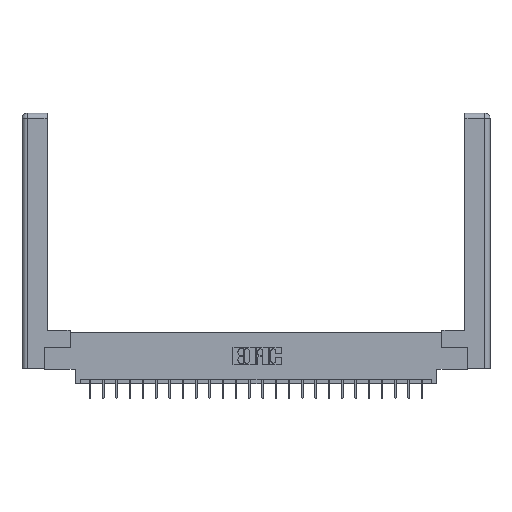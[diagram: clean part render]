
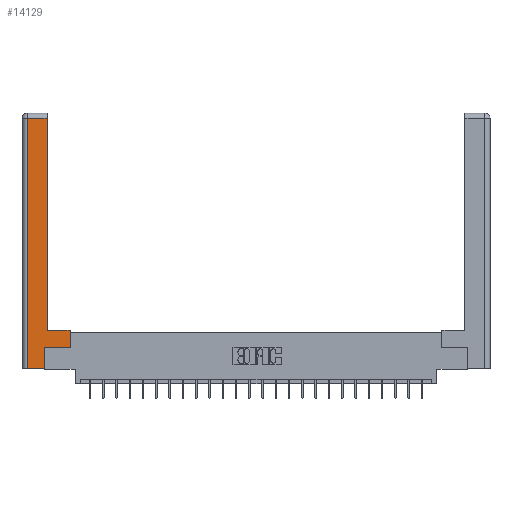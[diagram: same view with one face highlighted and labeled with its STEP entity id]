
A CAD part, top view. The second image highlights one B-rep face of the part: STEP entity #14129.
In plain terms, the highlighted planar face has unit normal (0, 0, 1).
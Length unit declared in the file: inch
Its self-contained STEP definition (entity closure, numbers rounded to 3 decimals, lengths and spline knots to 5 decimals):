
#980 = VERTEX_POINT ( 'NONE', #5465 ) ;
#1753 = CARTESIAN_POINT ( 'NONE',  ( 0.265, 0.245, 0. ) ) ;
#2010 = DIRECTION ( 'NONE',  ( 0., 1., 0. ) ) ;
#2089 = CARTESIAN_POINT ( 'NONE',  ( 0.265, 0.245, 0. ) ) ;
#2194 = LINE ( 'NONE', #23562, #3398 ) ;
#2288 = VERTEX_POINT ( 'NONE', #1753 ) ;
#2448 = DIRECTION ( 'NONE',  ( 1., 0., 0. ) ) ;
#2698 = LINE ( 'NONE', #21535, #18513 ) ;
#2741 = DIRECTION ( 'NONE',  ( 0., 0., -1. ) ) ;
#2962 = LINE ( 'NONE', #2089, #20273 ) ;
#3398 = VECTOR ( 'NONE', #2448, 39.37008 ) ;
#3611 = EDGE_CURVE ( 'NONE', #980, #16728, #10572, .T. ) ;
#3645 = ORIENTED_EDGE ( 'NONE', *, *, #22817, .T. ) ;
#3765 = ORIENTED_EDGE ( 'NONE', *, *, #8589, .T. ) ;
#4006 = LINE ( 'NONE', #23891, #23438 ) ;
#4472 = VECTOR ( 'NONE', #15790, 39.37008 ) ;
#5104 = ORIENTED_EDGE ( 'NONE', *, *, #24784, .T. ) ;
#5377 = EDGE_CURVE ( 'NONE', #16149, #980, #4006, .T. ) ;
#5465 = CARTESIAN_POINT ( 'NONE',  ( 0.295, 2.94, 0. ) ) ;
#5997 = CARTESIAN_POINT ( 'NONE',  ( 0.0615, 2.94, 0. ) ) ;
#6437 = CARTESIAN_POINT ( 'NONE',  ( 0., 0., 0. ) ) ;
#8413 = ORIENTED_EDGE ( 'NONE', *, *, #18346, .T. ) ;
#8589 = EDGE_CURVE ( 'NONE', #23346, #13900, #23147, .T. ) ;
#8873 = VECTOR ( 'NONE', #22036, 39.37008 ) ;
#10470 = DIRECTION ( 'NONE',  ( -1., 0., 0. ) ) ;
#10572 = LINE ( 'NONE', #5997, #4472 ) ;
#10596 = ORIENTED_EDGE ( 'NONE', *, *, #5377, .T. ) ;
#10843 = CARTESIAN_POINT ( 'NONE',  ( 0.295, 0.45, 0. ) ) ;
#11205 = EDGE_CURVE ( 'NONE', #2288, #22626, #2194, .T. ) ;
#11314 = DIRECTION ( 'NONE',  ( 0., -1., 0. ) ) ;
#11796 = VECTOR ( 'NONE', #11314, 39.37008 ) ;
#11833 = DIRECTION ( 'NONE',  ( 0., 1., 0. ) ) ;
#12417 = CARTESIAN_POINT ( 'NONE',  ( 0.265, 0., 0. ) ) ;
#12524 = ORIENTED_EDGE ( 'NONE', *, *, #14390, .T. ) ;
#13453 = CARTESIAN_POINT ( 'NONE',  ( 0.0615, 2.94, 0. ) ) ;
#13900 = VERTEX_POINT ( 'NONE', #23189 ) ;
#14129 = ADVANCED_FACE ( 'NONE', ( #18142 ), #16168, .F. ) ;
#14267 = DIRECTION ( 'NONE',  ( 0., 1., 0. ) ) ;
#14390 = EDGE_CURVE ( 'NONE', #13900, #2288, #2962, .T. ) ;
#14585 = AXIS2_PLACEMENT_3D ( 'NONE', #6437, #2741, #10470 ) ;
#14938 = EDGE_LOOP ( 'NONE', ( #10596, #19105, #5104, #3765, #12524, #23354, #8413, #3645 ) ) ;
#15790 = DIRECTION ( 'NONE',  ( -1., 0., 0. ) ) ;
#15851 = LINE ( 'NONE', #10843, #20388 ) ;
#16149 = VERTEX_POINT ( 'NONE', #21591 ) ;
#16168 = PLANE ( 'NONE',  #14585 ) ;
#16504 = VERTEX_POINT ( 'NONE', #24861 ) ;
#16609 = CARTESIAN_POINT ( 'NONE',  ( 0.565, 0.245, 0. ) ) ;
#16728 = VERTEX_POINT ( 'NONE', #13453 ) ;
#17296 = LINE ( 'NONE', #20960, #11796 ) ;
#18142 = FACE_OUTER_BOUND ( 'NONE', #14938, .T. ) ;
#18346 = EDGE_CURVE ( 'NONE', #22626, #16504, #2698, .T. ) ;
#18513 = VECTOR ( 'NONE', #11833, 39.37008 ) ;
#19105 = ORIENTED_EDGE ( 'NONE', *, *, #3611, .T. ) ;
#20273 = VECTOR ( 'NONE', #2010, 39.37008 ) ;
#20388 = VECTOR ( 'NONE', #20915, 39.37008 ) ;
#20554 = CARTESIAN_POINT ( 'NONE',  ( 0.0615, 0., 0. ) ) ;
#20915 = DIRECTION ( 'NONE',  ( -1., 0., 0. ) ) ;
#20960 = CARTESIAN_POINT ( 'NONE',  ( 0.0615, 0., 0. ) ) ;
#21535 = CARTESIAN_POINT ( 'NONE',  ( 0.565, 0.45, 0. ) ) ;
#21591 = CARTESIAN_POINT ( 'NONE',  ( 0.295, 0.45, 0. ) ) ;
#22036 = DIRECTION ( 'NONE',  ( 1., 0., 0. ) ) ;
#22626 = VERTEX_POINT ( 'NONE', #16609 ) ;
#22817 = EDGE_CURVE ( 'NONE', #16504, #16149, #15851, .T. ) ;
#23147 = LINE ( 'NONE', #12417, #8873 ) ;
#23189 = CARTESIAN_POINT ( 'NONE',  ( 0.265, 0., 0. ) ) ;
#23346 = VERTEX_POINT ( 'NONE', #20554 ) ;
#23354 = ORIENTED_EDGE ( 'NONE', *, *, #11205, .T. ) ;
#23438 = VECTOR ( 'NONE', #14267, 39.37008 ) ;
#23562 = CARTESIAN_POINT ( 'NONE',  ( 0.565, 0.245, 0. ) ) ;
#23891 = CARTESIAN_POINT ( 'NONE',  ( 0.295, 3., 0. ) ) ;
#24784 = EDGE_CURVE ( 'NONE', #16728, #23346, #17296, .T. ) ;
#24861 = CARTESIAN_POINT ( 'NONE',  ( 0.565, 0.45, 0. ) ) ;
